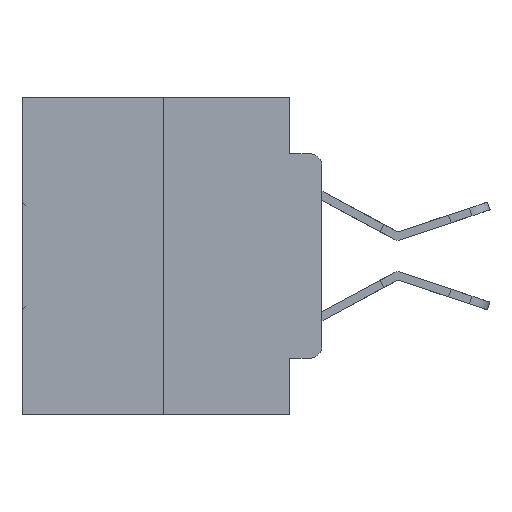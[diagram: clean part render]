
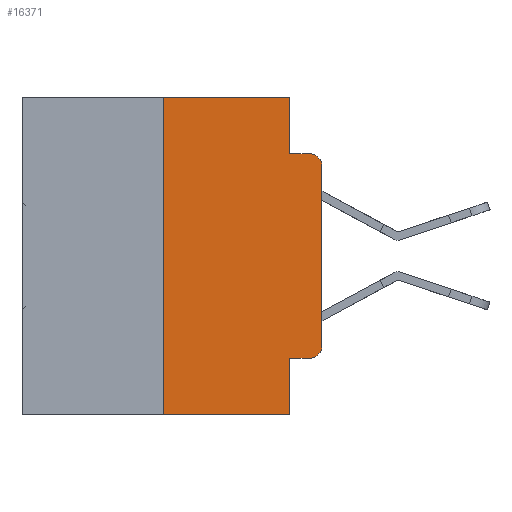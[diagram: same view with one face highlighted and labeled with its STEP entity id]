
A CAD part, left-side view. The second image highlights one B-rep face of the part: STEP entity #16371.
In plain terms, the highlighted planar face has unit normal (-1, 0, 0).
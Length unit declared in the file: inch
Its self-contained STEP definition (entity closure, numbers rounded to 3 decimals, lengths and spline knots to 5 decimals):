
#194 = PLANE ( 'NONE',  #734 ) ;
#249 = VECTOR ( 'NONE', #6318, 39.37008 ) ;
#734 = AXIS2_PLACEMENT_3D ( 'NONE', #5381, #22911, #7857 ) ;
#1193 = CARTESIAN_POINT ( 'NONE',  ( 0., 0.473, -0.5 ) ) ;
#2291 = VECTOR ( 'NONE', #20215, 39.37008 ) ;
#2412 = EDGE_CURVE ( 'NONE', #26041, #25158, #3094, .T. ) ;
#2640 = DIRECTION ( 'NONE',  ( 0., 0., 1. ) ) ;
#3094 = LINE ( 'NONE', #25280, #2291 ) ;
#3552 = ORIENTED_EDGE ( 'NONE', *, *, #11714, .F. ) ;
#3942 = ORIENTED_EDGE ( 'NONE', *, *, #20298, .T. ) ;
#4035 = CIRCLE ( 'NONE', #19439, 0.02 ) ;
#4130 = EDGE_CURVE ( 'NONE', #25158, #11520, #10877, .T. ) ;
#4240 = ORIENTED_EDGE ( 'NONE', *, *, #2412, .F. ) ;
#4411 = VERTEX_POINT ( 'NONE', #17930 ) ;
#4533 = DIRECTION ( 'NONE',  ( 0., -1., 0. ) ) ;
#5117 = VECTOR ( 'NONE', #27769, 39.37008 ) ;
#5381 = CARTESIAN_POINT ( 'NONE',  ( 0., 0.473, 0. ) ) ;
#5948 = VECTOR ( 'NONE', #2640, 39.37008 ) ;
#6156 = VERTEX_POINT ( 'NONE', #8546 ) ;
#6318 = DIRECTION ( 'NONE',  ( 0., -1., 0. ) ) ;
#6720 = LINE ( 'NONE', #15152, #5948 ) ;
#7320 = VECTOR ( 'NONE', #28978, 39.37008 ) ;
#7455 = DIRECTION ( 'NONE',  ( -1., 0., 0. ) ) ;
#7460 = EDGE_CURVE ( 'NONE', #4411, #11520, #4035, .T. ) ;
#7857 = DIRECTION ( 'NONE',  ( 0., 0., -1. ) ) ;
#8205 = FACE_OUTER_BOUND ( 'NONE', #20179, .T. ) ;
#8546 = CARTESIAN_POINT ( 'NONE',  ( 0., 0.25, 0. ) ) ;
#8585 = CARTESIAN_POINT ( 'NONE',  ( 0., 0.051, -0.4115 ) ) ;
#9150 = EDGE_CURVE ( 'NONE', #11212, #4411, #6720, .T. ) ;
#10877 = LINE ( 'NONE', #14413, #23432 ) ;
#11212 = VERTEX_POINT ( 'NONE', #12672 ) ;
#11520 = VERTEX_POINT ( 'NONE', #26561 ) ;
#11536 = VERTEX_POINT ( 'NONE', #31524 ) ;
#11573 = DIRECTION ( 'NONE',  ( -1., 0., 0. ) ) ;
#11589 = ORIENTED_EDGE ( 'NONE', *, *, #31553, .F. ) ;
#11652 = ORIENTED_EDGE ( 'NONE', *, *, #24937, .T. ) ;
#11714 = EDGE_CURVE ( 'NONE', #6156, #26041, #20643, .T. ) ;
#11981 = CARTESIAN_POINT ( 'NONE',  ( 0., 0.051, -0.4115 ) ) ;
#12672 = CARTESIAN_POINT ( 'NONE',  ( 0., 0., -0.3915 ) ) ;
#12751 = CARTESIAN_POINT ( 'NONE',  ( 0., 0.473, 0. ) ) ;
#13909 = CIRCLE ( 'NONE', #28061, 0.02 ) ;
#13955 = VECTOR ( 'NONE', #20304, 39.37008 ) ;
#13986 = LINE ( 'NONE', #13992, #7320 ) ;
#13992 = CARTESIAN_POINT ( 'NONE',  ( 0., 0.25, 0. ) ) ;
#14413 = CARTESIAN_POINT ( 'NONE',  ( 0., 0.051, -0.0885 ) ) ;
#15152 = CARTESIAN_POINT ( 'NONE',  ( 0., 0., 0. ) ) ;
#15619 = CARTESIAN_POINT ( 'NONE',  ( 0., 0.02, -0.4115 ) ) ;
#16371 = ADVANCED_FACE ( 'NONE', ( #8205 ), #194, .F. ) ;
#17516 = ORIENTED_EDGE ( 'NONE', *, *, #4130, .F. ) ;
#17930 = CARTESIAN_POINT ( 'NONE',  ( 0., 0., -0.1085 ) ) ;
#18589 = ORIENTED_EDGE ( 'NONE', *, *, #9150, .T. ) ;
#18938 = VERTEX_POINT ( 'NONE', #15619 ) ;
#19271 = ORIENTED_EDGE ( 'NONE', *, *, #7460, .T. ) ;
#19439 = AXIS2_PLACEMENT_3D ( 'NONE', #26581, #11573, #29061 ) ;
#20179 = EDGE_LOOP ( 'NONE', ( #18589, #19271, #17516, #4240, #3552, #11589, #3942, #20619, #20261, #11652 ) ) ;
#20215 = DIRECTION ( 'NONE',  ( 0., 0., -1. ) ) ;
#20261 = ORIENTED_EDGE ( 'NONE', *, *, #26589, .T. ) ;
#20298 = EDGE_CURVE ( 'NONE', #11536, #25148, #20379, .T. ) ;
#20304 = DIRECTION ( 'NONE',  ( 0., -1., 0. ) ) ;
#20379 = LINE ( 'NONE', #1193, #249 ) ;
#20619 = ORIENTED_EDGE ( 'NONE', *, *, #29893, .F. ) ;
#20643 = LINE ( 'NONE', #12751, #13955 ) ;
#20931 = CARTESIAN_POINT ( 'NONE',  ( 0., 0.051, -0.0885 ) ) ;
#22062 = VERTEX_POINT ( 'NONE', #8585 ) ;
#22495 = CARTESIAN_POINT ( 'NONE',  ( 0., 0.02, -0.3915 ) ) ;
#22911 = DIRECTION ( 'NONE',  ( 1., 0., 0. ) ) ;
#23432 = VECTOR ( 'NONE', #29494, 39.37008 ) ;
#23620 = VECTOR ( 'NONE', #4533, 39.37008 ) ;
#24937 = EDGE_CURVE ( 'NONE', #18938, #11212, #13909, .T. ) ;
#25041 = DIRECTION ( 'NONE',  ( 0., 0., -1. ) ) ;
#25135 = LINE ( 'NONE', #25296, #5117 ) ;
#25148 = VERTEX_POINT ( 'NONE', #30940 ) ;
#25158 = VERTEX_POINT ( 'NONE', #20931 ) ;
#25280 = CARTESIAN_POINT ( 'NONE',  ( 0., 0.051, 0. ) ) ;
#25296 = CARTESIAN_POINT ( 'NONE',  ( 0., 0.051, 0. ) ) ;
#25996 = LINE ( 'NONE', #11981, #23620 ) ;
#26041 = VERTEX_POINT ( 'NONE', #27221 ) ;
#26561 = CARTESIAN_POINT ( 'NONE',  ( 0., 0.02, -0.0885 ) ) ;
#26581 = CARTESIAN_POINT ( 'NONE',  ( 0., 0.02, -0.1085 ) ) ;
#26589 = EDGE_CURVE ( 'NONE', #22062, #18938, #25996, .T. ) ;
#27221 = CARTESIAN_POINT ( 'NONE',  ( 0., 0.051, 0. ) ) ;
#27769 = DIRECTION ( 'NONE',  ( 0., 0., -1. ) ) ;
#28061 = AXIS2_PLACEMENT_3D ( 'NONE', #22495, #7455, #25041 ) ;
#28978 = DIRECTION ( 'NONE',  ( 0., 0., 1. ) ) ;
#29061 = DIRECTION ( 'NONE',  ( 0., 0., -1. ) ) ;
#29494 = DIRECTION ( 'NONE',  ( 0., -1., 0. ) ) ;
#29893 = EDGE_CURVE ( 'NONE', #22062, #25148, #25135, .T. ) ;
#30940 = CARTESIAN_POINT ( 'NONE',  ( 0., 0.051, -0.5 ) ) ;
#31524 = CARTESIAN_POINT ( 'NONE',  ( 0., 0.25, -0.5 ) ) ;
#31553 = EDGE_CURVE ( 'NONE', #11536, #6156, #13986, .T. ) ;
